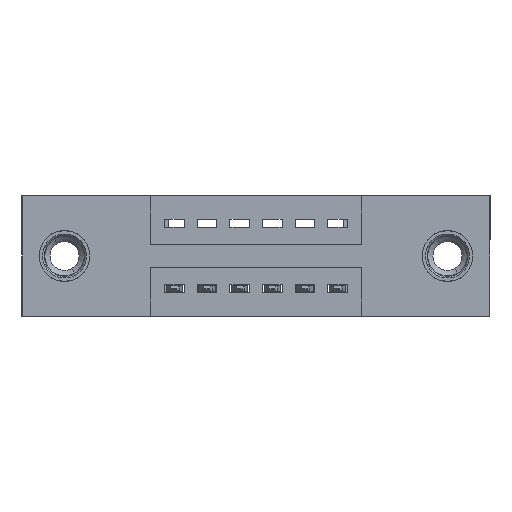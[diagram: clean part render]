
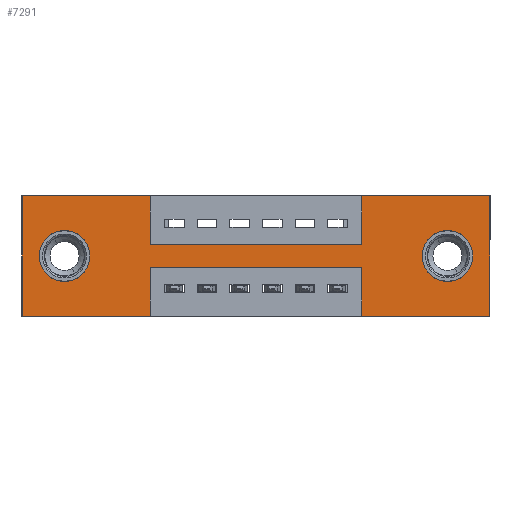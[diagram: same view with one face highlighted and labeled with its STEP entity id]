
A CAD part, front view. The second image highlights one B-rep face of the part: STEP entity #7291.
In plain terms, the highlighted planar face has unit normal (0, -1, 0).
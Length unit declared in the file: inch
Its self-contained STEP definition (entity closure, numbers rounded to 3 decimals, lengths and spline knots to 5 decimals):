
#179 = ORIENTED_EDGE ( 'NONE', *, *, #10138, .T. ) ;
#206 = EDGE_CURVE ( 'NONE', #11216, #5154, #5123, .T. ) ;
#233 = EDGE_CURVE ( 'NONE', #9246, #2212, #6238, .T. ) ;
#341 = ORIENTED_EDGE ( 'NONE', *, *, #8692, .F. ) ;
#365 = VECTOR ( 'NONE', #2793, 39.37008 ) ;
#413 = FACE_BOUND ( 'NONE', #3893, .T. ) ;
#585 = EDGE_CURVE ( 'NONE', #10567, #6690, #9088, .T. ) ;
#598 = DIRECTION ( 'NONE',  ( 0., 0., 1. ) ) ;
#823 = AXIS2_PLACEMENT_3D ( 'NONE', #10186, #6408, #7368 ) ;
#1129 = ORIENTED_EDGE ( 'NONE', *, *, #3568, .F. ) ;
#1351 = EDGE_CURVE ( 'NONE', #9087, #11216, #8939, .T. ) ;
#1526 = CARTESIAN_POINT ( 'NONE',  ( 1.0425, 0., -0.22 ) ) ;
#1656 = CARTESIAN_POINT ( 'NONE',  ( 0.3925, 0., -0.37 ) ) ;
#1751 = CARTESIAN_POINT ( 'NONE',  ( 1.435, 0., -0.37 ) ) ;
#1842 = EDGE_CURVE ( 'NONE', #4910, #8098, #11583, .T. ) ;
#1869 = AXIS2_PLACEMENT_3D ( 'NONE', #4397, #5419, #8907 ) ;
#1873 = LINE ( 'NONE', #9457, #10863 ) ;
#2212 = VERTEX_POINT ( 'NONE', #3135 ) ;
#2248 = EDGE_CURVE ( 'NONE', #6690, #3935, #3122, .T. ) ;
#2264 = EDGE_CURVE ( 'NONE', #11400, #9436, #1873, .T. ) ;
#2383 = DIRECTION ( 'NONE',  ( -1., 0., 0. ) ) ;
#2417 = DIRECTION ( 'NONE',  ( 1., 0., 0. ) ) ;
#2437 = LINE ( 'NONE', #4310, #6908 ) ;
#2793 = DIRECTION ( 'NONE',  ( 1., 0., 0. ) ) ;
#3066 = ORIENTED_EDGE ( 'NONE', *, *, #585, .F. ) ;
#3069 = CARTESIAN_POINT ( 'NONE',  ( 0., 0., -0.37 ) ) ;
#3122 = LINE ( 'NONE', #11392, #5086 ) ;
#3135 = CARTESIAN_POINT ( 'NONE',  ( 0.13, 0., -0.107 ) ) ;
#3289 = VECTOR ( 'NONE', #7679, 39.37008 ) ;
#3320 = DIRECTION ( 'NONE',  ( -1., 0., 0. ) ) ;
#3568 = EDGE_CURVE ( 'NONE', #5324, #8181, #4211, .T. ) ;
#3769 = DIRECTION ( 'NONE',  ( 0., 1., 0. ) ) ;
#3847 = DIRECTION ( 'NONE',  ( 0., 0., -1. ) ) ;
#3893 = EDGE_LOOP ( 'NONE', ( #4840, #3996 ) ) ;
#3935 = VERTEX_POINT ( 'NONE', #1526 ) ;
#3944 = EDGE_LOOP ( 'NONE', ( #11547, #11594, #4911, #3066, #341, #1129, #4010, #8026, #9333, #5302, #11224, #4295 ) ) ;
#3968 = EDGE_CURVE ( 'NONE', #11138, #7184, #10548, .T. ) ;
#3996 = ORIENTED_EDGE ( 'NONE', *, *, #233, .T. ) ;
#4010 = ORIENTED_EDGE ( 'NONE', *, *, #4434, .F. ) ;
#4033 = EDGE_CURVE ( 'NONE', #2212, #9246, #9292, .T. ) ;
#4037 = DIRECTION ( 'NONE',  ( -1., 0., 0. ) ) ;
#4075 = AXIS2_PLACEMENT_3D ( 'NONE', #7203, #3769, #5404 ) ;
#4153 = DIRECTION ( 'NONE',  ( 0., 0., 1. ) ) ;
#4196 = DIRECTION ( 'NONE',  ( 0., -1., 0. ) ) ;
#4211 = LINE ( 'NONE', #4668, #7304 ) ;
#4271 = EDGE_CURVE ( 'NONE', #3935, #11138, #5603, .T. ) ;
#4295 = ORIENTED_EDGE ( 'NONE', *, *, #4659, .F. ) ;
#4310 = CARTESIAN_POINT ( 'NONE',  ( 1.0425, 0., 0. ) ) ;
#4397 = CARTESIAN_POINT ( 'NONE',  ( 1.305, 0., -0.185 ) ) ;
#4434 = EDGE_CURVE ( 'NONE', #5154, #5324, #2437, .T. ) ;
#4659 = EDGE_CURVE ( 'NONE', #7184, #11400, #10865, .T. ) ;
#4668 = CARTESIAN_POINT ( 'NONE',  ( 0., 0., 0. ) ) ;
#4679 = CARTESIAN_POINT ( 'NONE',  ( 0., 0., 0. ) ) ;
#4840 = ORIENTED_EDGE ( 'NONE', *, *, #4033, .T. ) ;
#4910 = VERTEX_POINT ( 'NONE', #8176 ) ;
#4911 = ORIENTED_EDGE ( 'NONE', *, *, #2248, .F. ) ;
#5005 = CARTESIAN_POINT ( 'NONE',  ( 0.13, 0., -0.263 ) ) ;
#5086 = VECTOR ( 'NONE', #598, 39.37008 ) ;
#5094 = CARTESIAN_POINT ( 'NONE',  ( 0.3925, 0., -0.37 ) ) ;
#5123 = LINE ( 'NONE', #10072, #365 ) ;
#5154 = VERTEX_POINT ( 'NONE', #8238 ) ;
#5302 = ORIENTED_EDGE ( 'NONE', *, *, #10382, .F. ) ;
#5324 = VERTEX_POINT ( 'NONE', #7201 ) ;
#5329 = VECTOR ( 'NONE', #2383, 39.37008 ) ;
#5404 = DIRECTION ( 'NONE',  ( 0., 0., 1. ) ) ;
#5419 = DIRECTION ( 'NONE',  ( 0., 1., 0. ) ) ;
#5461 = CARTESIAN_POINT ( 'NONE',  ( 0.3925, 0., -0.22 ) ) ;
#5562 = VECTOR ( 'NONE', #11574, 39.37008 ) ;
#5603 = LINE ( 'NONE', #10420, #5329 ) ;
#5972 = DIRECTION ( 'NONE',  ( 0., 0., -1. ) ) ;
#6140 = FACE_BOUND ( 'NONE', #10869, .T. ) ;
#6179 = CARTESIAN_POINT ( 'NONE',  ( 1.435, 0., 0. ) ) ;
#6238 = CIRCLE ( 'NONE', #4075, 0.078 ) ;
#6408 = DIRECTION ( 'NONE',  ( 0., 1., 0. ) ) ;
#6675 = CARTESIAN_POINT ( 'NONE',  ( 0., 0., -0.37 ) ) ;
#6684 = ORIENTED_EDGE ( 'NONE', *, *, #1842, .T. ) ;
#6690 = VERTEX_POINT ( 'NONE', #7431 ) ;
#6908 = VECTOR ( 'NONE', #11467, 39.37008 ) ;
#6982 = CARTESIAN_POINT ( 'NONE',  ( 0., 0., 0. ) ) ;
#6992 = VECTOR ( 'NONE', #5972, 39.37008 ) ;
#7184 = VERTEX_POINT ( 'NONE', #1656 ) ;
#7193 = CARTESIAN_POINT ( 'NONE',  ( 0.3925, 0., 0. ) ) ;
#7201 = CARTESIAN_POINT ( 'NONE',  ( 1.0425, 0., 0. ) ) ;
#7203 = CARTESIAN_POINT ( 'NONE',  ( 0.13, 0., -0.185 ) ) ;
#7291 = ADVANCED_FACE ( 'NONE', ( #6140, #413, #9831 ), #8685, .T. ) ;
#7304 = VECTOR ( 'NONE', #10997, 39.37008 ) ;
#7368 = DIRECTION ( 'NONE',  ( 0., 0., 1. ) ) ;
#7431 = CARTESIAN_POINT ( 'NONE',  ( 1.0425, 0., -0.37 ) ) ;
#7679 = DIRECTION ( 'NONE',  ( 0., 0., -1. ) ) ;
#7772 = AXIS2_PLACEMENT_3D ( 'NONE', #9583, #4196, #7809 ) ;
#7809 = DIRECTION ( 'NONE',  ( 0., 0., -1. ) ) ;
#7962 = LINE ( 'NONE', #6179, #5562 ) ;
#8026 = ORIENTED_EDGE ( 'NONE', *, *, #206, .F. ) ;
#8090 = CARTESIAN_POINT ( 'NONE',  ( 1.435, 0., 0. ) ) ;
#8098 = VERTEX_POINT ( 'NONE', #10560 ) ;
#8171 = AXIS2_PLACEMENT_3D ( 'NONE', #8330, #11121, #3847 ) ;
#8176 = CARTESIAN_POINT ( 'NONE',  ( 1.305, 0., -0.107 ) ) ;
#8181 = VERTEX_POINT ( 'NONE', #8090 ) ;
#8224 = CARTESIAN_POINT ( 'NONE',  ( 0.3925, 0., -0.15 ) ) ;
#8238 = CARTESIAN_POINT ( 'NONE',  ( 1.0425, 0., -0.15 ) ) ;
#8330 = CARTESIAN_POINT ( 'NONE',  ( 1.305, 0., -0.185 ) ) ;
#8624 = VECTOR ( 'NONE', #4037, 39.37008 ) ;
#8685 = PLANE ( 'NONE',  #7772 ) ;
#8692 = EDGE_CURVE ( 'NONE', #8181, #10567, #7962, .T. ) ;
#8750 = CARTESIAN_POINT ( 'NONE',  ( 0., 0., -0.37 ) ) ;
#8803 = VECTOR ( 'NONE', #3320, 39.37008 ) ;
#8907 = DIRECTION ( 'NONE',  ( 0., 0., -1. ) ) ;
#8939 = LINE ( 'NONE', #9482, #3289 ) ;
#9087 = VERTEX_POINT ( 'NONE', #7193 ) ;
#9088 = LINE ( 'NONE', #8750, #8803 ) ;
#9246 = VERTEX_POINT ( 'NONE', #5005 ) ;
#9292 = CIRCLE ( 'NONE', #823, 0.078 ) ;
#9333 = ORIENTED_EDGE ( 'NONE', *, *, #1351, .F. ) ;
#9436 = VERTEX_POINT ( 'NONE', #4679 ) ;
#9457 = CARTESIAN_POINT ( 'NONE',  ( 0., 0., 0. ) ) ;
#9482 = CARTESIAN_POINT ( 'NONE',  ( 0.3925, 0., 0. ) ) ;
#9583 = CARTESIAN_POINT ( 'NONE',  ( 0., 0., -0.37 ) ) ;
#9831 = FACE_OUTER_BOUND ( 'NONE', #3944, .T. ) ;
#9902 = LINE ( 'NONE', #6982, #10056 ) ;
#10056 = VECTOR ( 'NONE', #2417, 39.37008 ) ;
#10072 = CARTESIAN_POINT ( 'NONE',  ( 0.3925, 0., -0.15 ) ) ;
#10138 = EDGE_CURVE ( 'NONE', #8098, #4910, #11169, .T. ) ;
#10186 = CARTESIAN_POINT ( 'NONE',  ( 0.13, 0., -0.185 ) ) ;
#10382 = EDGE_CURVE ( 'NONE', #9436, #9087, #9902, .T. ) ;
#10420 = CARTESIAN_POINT ( 'NONE',  ( 0.3925, 0., -0.22 ) ) ;
#10548 = LINE ( 'NONE', #5094, #6992 ) ;
#10560 = CARTESIAN_POINT ( 'NONE',  ( 1.305, 0., -0.263 ) ) ;
#10567 = VERTEX_POINT ( 'NONE', #1751 ) ;
#10863 = VECTOR ( 'NONE', #4153, 39.37008 ) ;
#10865 = LINE ( 'NONE', #6675, #8624 ) ;
#10869 = EDGE_LOOP ( 'NONE', ( #6684, #179 ) ) ;
#10997 = DIRECTION ( 'NONE',  ( 1., 0., 0. ) ) ;
#11121 = DIRECTION ( 'NONE',  ( 0., 1., 0. ) ) ;
#11138 = VERTEX_POINT ( 'NONE', #5461 ) ;
#11169 = CIRCLE ( 'NONE', #8171, 0.078 ) ;
#11216 = VERTEX_POINT ( 'NONE', #8224 ) ;
#11224 = ORIENTED_EDGE ( 'NONE', *, *, #2264, .F. ) ;
#11392 = CARTESIAN_POINT ( 'NONE',  ( 1.0425, 0., -0.37 ) ) ;
#11400 = VERTEX_POINT ( 'NONE', #3069 ) ;
#11467 = DIRECTION ( 'NONE',  ( 0., 0., 1. ) ) ;
#11547 = ORIENTED_EDGE ( 'NONE', *, *, #3968, .F. ) ;
#11574 = DIRECTION ( 'NONE',  ( 0., 0., -1. ) ) ;
#11583 = CIRCLE ( 'NONE', #1869, 0.078 ) ;
#11594 = ORIENTED_EDGE ( 'NONE', *, *, #4271, .F. ) ;
